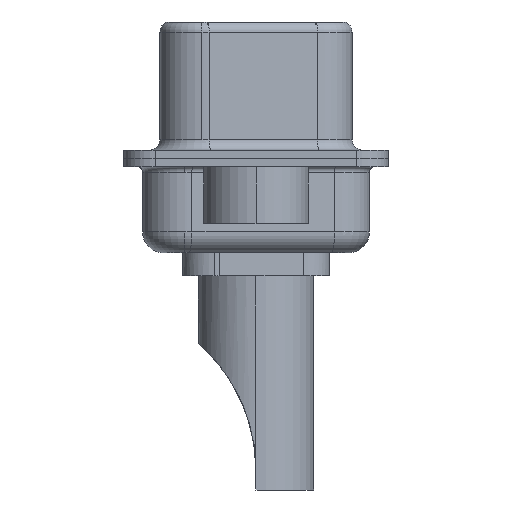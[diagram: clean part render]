
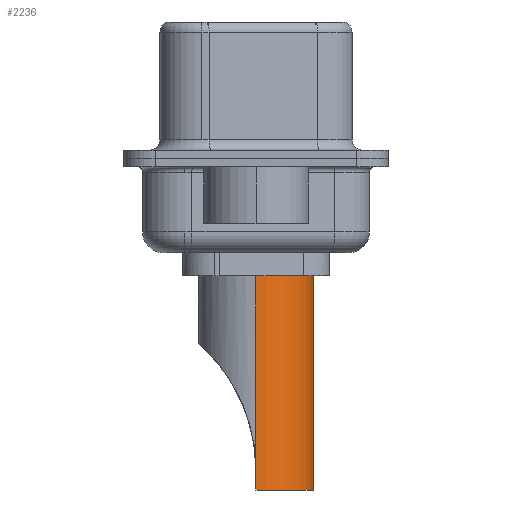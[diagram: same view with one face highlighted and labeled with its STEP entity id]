
A CAD part, left-side view. The second image highlights one B-rep face of the part: STEP entity #2236.
In plain terms, the highlighted cylindrical face has radius 2.75 mm (diameter 5.5 mm), a partial arc.
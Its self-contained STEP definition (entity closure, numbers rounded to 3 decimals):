
#74 = EDGE_CURVE ( 'NONE', #2005, #10865, #11391, .T. ) ;
#808 = DIRECTION ( 'NONE',  ( 0., 0., 1. ) ) ;
#1421 = LINE ( 'NONE', #7411, #14317 ) ;
#1942 = EDGE_CURVE ( 'NONE', #8970, #10865, #1421, .T. ) ;
#2005 = VERTEX_POINT ( 'NONE', #10232 ) ;
#2236 = ADVANCED_FACE ( 'NONE', ( #4152 ), #10369, .T. ) ;
#2346 = LINE ( 'NONE', #10769, #5865 ) ;
#2470 = EDGE_LOOP ( 'NONE', ( #6783, #5906, #5971, #8816, #12604, #4699 ) ) ;
#2522 = DIRECTION ( 'NONE',  ( 0., 0., -1. ) ) ;
#2688 = DIRECTION ( 'NONE',  ( 0., 0., 1. ) ) ;
#3039 = LINE ( 'NONE', #7155, #8494 ) ;
#4069 = VERTEX_POINT ( 'NONE', #9242 ) ;
#4079 = CARTESIAN_POINT ( 'NONE',  ( 0., 0., 4.234 ) ) ;
#4152 = FACE_OUTER_BOUND ( 'NONE', #2470, .T. ) ;
#4286 = DIRECTION ( 'NONE',  ( 0., 0., 1. ) ) ;
#4693 = DIRECTION ( 'NONE',  ( 0., 0., -1. ) ) ;
#4699 = ORIENTED_EDGE ( 'NONE', *, *, #5982, .F. ) ;
#5200 = DIRECTION ( 'NONE',  ( 1., 0., 0. ) ) ;
#5542 = CARTESIAN_POINT ( 'NONE',  ( -2.75, 0., 4.234 ) ) ;
#5865 = VECTOR ( 'NONE', #808, 1000. ) ;
#5906 = ORIENTED_EDGE ( 'NONE', *, *, #9287, .T. ) ;
#5971 = ORIENTED_EDGE ( 'NONE', *, *, #74, .T. ) ;
#5982 = EDGE_CURVE ( 'NONE', #4069, #12126, #6815, .T. ) ;
#6065 = VERTEX_POINT ( 'NONE', #13672 ) ;
#6783 = ORIENTED_EDGE ( 'NONE', *, *, #14972, .F. ) ;
#6815 = CIRCLE ( 'NONE', #10523, 2.75 ) ;
#7090 = CARTESIAN_POINT ( 'NONE',  ( 2.75, 0., 1.5 ) ) ;
#7155 = CARTESIAN_POINT ( 'NONE',  ( -2.75, 0., -8.7 ) ) ;
#7240 = AXIS2_PLACEMENT_3D ( 'NONE', #12328, #9822, #13449 ) ;
#7411 = CARTESIAN_POINT ( 'NONE',  ( 2.75, 0., -8.7 ) ) ;
#8494 = VECTOR ( 'NONE', #4693, 1000. ) ;
#8816 = ORIENTED_EDGE ( 'NONE', *, *, #1942, .F. ) ;
#8970 = VERTEX_POINT ( 'NONE', #10319 ) ;
#9180 = LINE ( 'NONE', #5542, #9570 ) ;
#9242 = CARTESIAN_POINT ( 'NONE',  ( -2.75, 0., 1.5 ) ) ;
#9287 = EDGE_CURVE ( 'NONE', #6065, #2005, #3039, .T. ) ;
#9570 = VECTOR ( 'NONE', #4286, 1000. ) ;
#9634 = EDGE_CURVE ( 'NONE', #8970, #12126, #2346, .T. ) ;
#9822 = DIRECTION ( 'NONE',  ( 0., 0., 1. ) ) ;
#10232 = CARTESIAN_POINT ( 'NONE',  ( -2.75, 0., -8.7 ) ) ;
#10319 = CARTESIAN_POINT ( 'NONE',  ( 2.75, 0., -7.764 ) ) ;
#10369 = CYLINDRICAL_SURFACE ( 'NONE', #10602, 2.75 ) ;
#10523 = AXIS2_PLACEMENT_3D ( 'NONE', #13855, #2688, #5200 ) ;
#10602 = AXIS2_PLACEMENT_3D ( 'NONE', #4079, #15316, #12610 ) ;
#10769 = CARTESIAN_POINT ( 'NONE',  ( 2.75, 0., 4.234 ) ) ;
#10865 = VERTEX_POINT ( 'NONE', #14232 ) ;
#11391 = CIRCLE ( 'NONE', #7240, 2.75 ) ;
#12126 = VERTEX_POINT ( 'NONE', #7090 ) ;
#12328 = CARTESIAN_POINT ( 'NONE',  ( 0., 0., -8.7 ) ) ;
#12604 = ORIENTED_EDGE ( 'NONE', *, *, #9634, .T. ) ;
#12610 = DIRECTION ( 'NONE',  ( 1., 0., 0. ) ) ;
#13449 = DIRECTION ( 'NONE',  ( 1., 0., 0. ) ) ;
#13672 = CARTESIAN_POINT ( 'NONE',  ( -2.75, 0., -7.764 ) ) ;
#13855 = CARTESIAN_POINT ( 'NONE',  ( 0., 0., 1.5 ) ) ;
#14232 = CARTESIAN_POINT ( 'NONE',  ( 2.75, 0., -8.7 ) ) ;
#14317 = VECTOR ( 'NONE', #2522, 1000. ) ;
#14972 = EDGE_CURVE ( 'NONE', #6065, #4069, #9180, .T. ) ;
#15316 = DIRECTION ( 'NONE',  ( 0., 0., 1. ) ) ;
